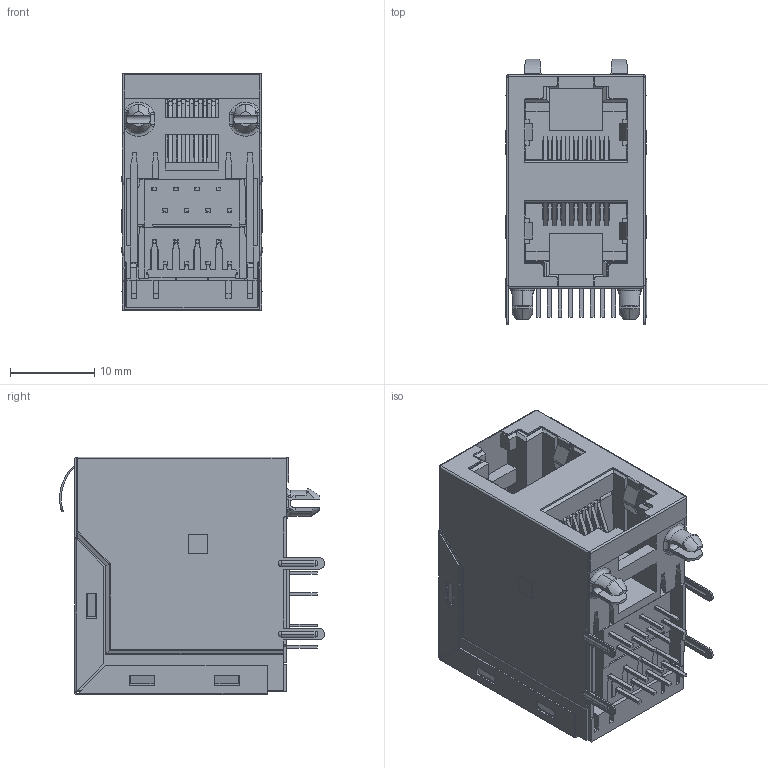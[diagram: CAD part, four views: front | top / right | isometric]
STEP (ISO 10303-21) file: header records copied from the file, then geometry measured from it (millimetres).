
FILE_DESCRIPTION (( 'STEP AP203' ), '1' );
FILE_NAME ('J96028822N00221.STEP', '2020-03-20T22:48:05', ( '' ), ( '' ), 'SwSTEP 2.0', 'SolidWorks 2016', '' );
FILE_SCHEMA (( 'CONFIG_CONTROL_DESIGN' ));
Length unit declared in the file: millimetre
Products named in the file (10): 96 Insulator Insert; 96 Grounding_2 Ports; 96 Back Plate_2 Ports; 96 Shield_2 Ports No LED - EMI; 96 Contacts Lower; 96 Contact Lock Upper; 96 Insulator_2 Ports; J96028822N00221; 96 Contact Lock Lower; 96 Contacts Upper
Assembly tree (9 placements, depth 2):
  J96028822N00221
    96 Insulator_2 Ports
    96 Contacts Lower
    96 Contact Lock Lower
    96 Grounding_2 Ports
    96 Contacts Upper
    96 Contact Lock Upper
    96 Insulator Insert
    96 Back Plate_2 Ports
    96 Shield_2 Ports No LED - EMI
Bounding box: 16.8 x 31.38 x 28.15 mm (x, y, z)
Volume: 6698.2 mm3; surface area: 18464.9 mm2
Topology: 23 solids, 23 shells, 2301 faces, 6450 edges, 4135 vertices
Faces by surface type: plane 1781, cylinder 414, bspline 98, cone 8
Entity records: 76202 total; most frequent: CARTESIAN_POINT 17069, ORIENTED_EDGE 12868, DIRECTION 10938, EDGE_CURVE 6434, LINE 5234, VECTOR 5234, VERTEX_POINT 4135, AXIS2_PLACEMENT_3D 2852
